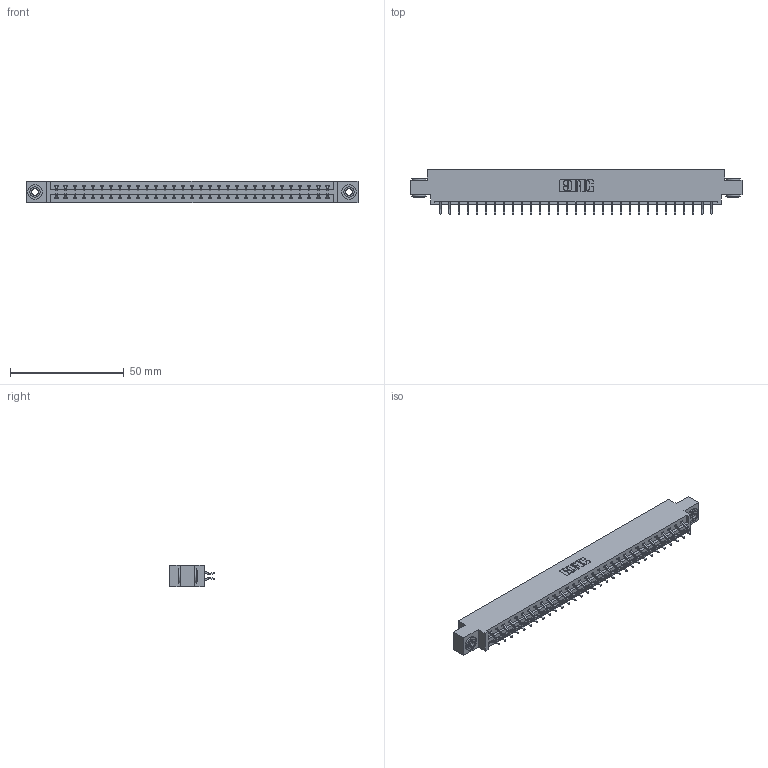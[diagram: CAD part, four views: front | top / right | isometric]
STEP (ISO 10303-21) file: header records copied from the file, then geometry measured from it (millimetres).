
FILE_DESCRIPTION (( 'STEP AP203' ), '1' );
FILE_NAME ('337-062-556-803.STEP', '2018-08-11T04:44:31', ( '' ), ( '' ), 'SwSTEP 2.0', 'SolidWorks 2016', '' );
FILE_SCHEMA (( 'CONFIG_CONTROL_DESIGN' ));
Length unit declared in the file: inch
Products named in the file (4): 345-250-002_345-250-002-102; 337-062-556-803; 337 Part_0.170 Offset - 0.156 Dia-TH; 345-292-001_556 Tail
Assembly tree (65 placements, depth 2):
  337-062-556-803
    337 Part_0.170 Offset - 0.156 Dia-TH
    345-292-001_556 Tail  x62
    345-250-002_345-250-002-102  x2
Bounding box: 145.85 x 19.57 x 9.4 mm (x, y, z)
Volume: 15123.5 mm3; surface area: 17257.1 mm2
Topology: 65 solids, 65 shells, 3876 faces, 11497 edges, 7578 vertices
Faces by surface type: plane 2688, cylinder 1180, cone 8
Entity records: 26460 total; most frequent: CARTESIAN_POINT 4457, ORIENTED_EDGE 4374, DIRECTION 3833, EDGE_CURVE 2187, LINE 2027, VECTOR 2027, VERTEX_POINT 1454, AXIS2_PLACEMENT_3D 903
